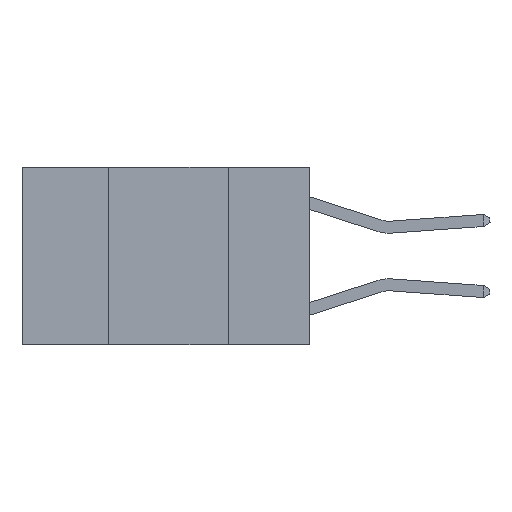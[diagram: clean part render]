
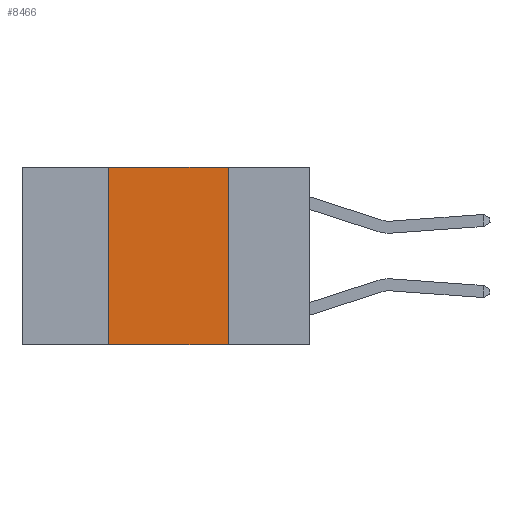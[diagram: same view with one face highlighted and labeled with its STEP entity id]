
A CAD part, left-side view. The second image highlights one B-rep face of the part: STEP entity #8466.
In plain terms, the highlighted planar face has unit normal (-1, 0, 0).
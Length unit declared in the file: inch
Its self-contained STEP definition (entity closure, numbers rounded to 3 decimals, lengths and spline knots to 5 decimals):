
#74 = EDGE_CURVE ( 'NONE', #1799, #5439, #8786, .T. ) ;
#178 = VECTOR ( 'NONE', #7466, 39.37008 ) ;
#194 = DIRECTION ( 'NONE',  ( 0., 0., 1. ) ) ;
#370 = CARTESIAN_POINT ( 'NONE',  ( 0., 0.42, -0.37 ) ) ;
#1058 = CARTESIAN_POINT ( 'NONE',  ( 0., 0.42, 0. ) ) ;
#1095 = EDGE_CURVE ( 'NONE', #3699, #1799, #8657, .T. ) ;
#1184 = ORIENTED_EDGE ( 'NONE', *, *, #1095, .F. ) ;
#1555 = DIRECTION ( 'NONE',  ( 0., 0., -1. ) ) ;
#1799 = VERTEX_POINT ( 'NONE', #8999 ) ;
#2082 = VERTEX_POINT ( 'NONE', #370 ) ;
#2159 = AXIS2_PLACEMENT_3D ( 'NONE', #10294, #2235, #7966 ) ;
#2235 = DIRECTION ( 'NONE',  ( 1., 0., 0. ) ) ;
#2274 = VECTOR ( 'NONE', #1555, 39.37008 ) ;
#2286 = CARTESIAN_POINT ( 'NONE',  ( 0., 0.17, -0.37 ) ) ;
#3137 = EDGE_LOOP ( 'NONE', ( #6806, #1184, #3626, #7971 ) ) ;
#3455 = EDGE_CURVE ( 'NONE', #2082, #5439, #6050, .T. ) ;
#3533 = LINE ( 'NONE', #1058, #5480 ) ;
#3626 = ORIENTED_EDGE ( 'NONE', *, *, #5802, .F. ) ;
#3665 = CARTESIAN_POINT ( 'NONE',  ( 0., 0.17, 0. ) ) ;
#3699 = VERTEX_POINT ( 'NONE', #7459 ) ;
#3771 = DIRECTION ( 'NONE',  ( 0., -1., 0. ) ) ;
#5439 = VERTEX_POINT ( 'NONE', #2286 ) ;
#5480 = VECTOR ( 'NONE', #194, 39.37008 ) ;
#5802 = EDGE_CURVE ( 'NONE', #2082, #3699, #3533, .T. ) ;
#6050 = LINE ( 'NONE', #7018, #7926 ) ;
#6476 = FACE_OUTER_BOUND ( 'NONE', #3137, .T. ) ;
#6737 = CARTESIAN_POINT ( 'NONE',  ( 0., 0.6, 0. ) ) ;
#6806 = ORIENTED_EDGE ( 'NONE', *, *, #74, .F. ) ;
#7018 = CARTESIAN_POINT ( 'NONE',  ( 0., 0.6, -0.37 ) ) ;
#7154 = PLANE ( 'NONE',  #2159 ) ;
#7459 = CARTESIAN_POINT ( 'NONE',  ( 0., 0.42, 0. ) ) ;
#7466 = DIRECTION ( 'NONE',  ( 0., -1., 0. ) ) ;
#7926 = VECTOR ( 'NONE', #3771, 39.37008 ) ;
#7966 = DIRECTION ( 'NONE',  ( 0., 0., -1. ) ) ;
#7971 = ORIENTED_EDGE ( 'NONE', *, *, #3455, .T. ) ;
#8466 = ADVANCED_FACE ( 'NONE', ( #6476 ), #7154, .F. ) ;
#8657 = LINE ( 'NONE', #6737, #178 ) ;
#8786 = LINE ( 'NONE', #3665, #2274 ) ;
#8999 = CARTESIAN_POINT ( 'NONE',  ( 0., 0.17, 0. ) ) ;
#10294 = CARTESIAN_POINT ( 'NONE',  ( 0., 0.6, 0. ) ) ;
